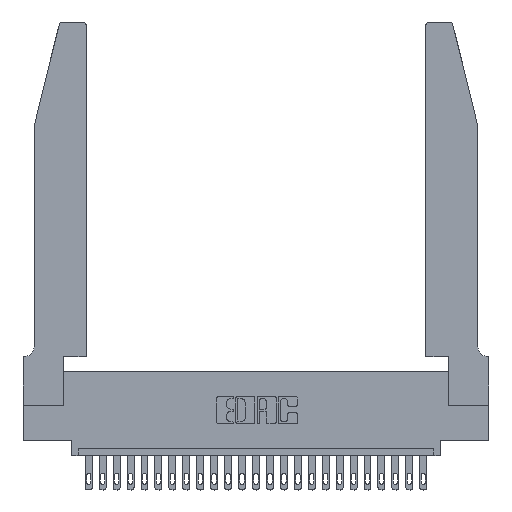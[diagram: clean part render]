
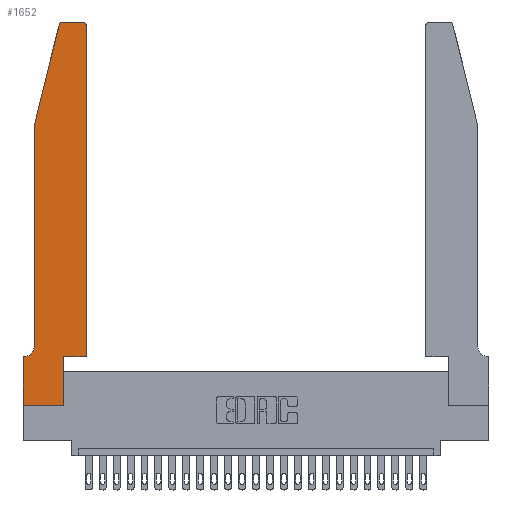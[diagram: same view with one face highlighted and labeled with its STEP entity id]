
A CAD part, top view. The second image highlights one B-rep face of the part: STEP entity #1652.
In plain terms, the highlighted planar face has unit normal (0, 0, 1).
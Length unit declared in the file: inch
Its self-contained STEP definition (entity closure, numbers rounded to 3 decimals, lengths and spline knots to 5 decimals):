
#261 = CIRCLE ( 'NONE', #6762, 0.03 ) ;
#821 = EDGE_CURVE ( 'NONE', #6447, #13358, #22657, .T. ) ;
#1014 = DIRECTION ( 'NONE',  ( 0., 0., 1. ) ) ;
#1505 = VECTOR ( 'NONE', #7983, 39.37008 ) ;
#1580 = CIRCLE ( 'NONE', #14817, 0.03 ) ;
#1652 = ADVANCED_FACE ( 'NONE', ( #4188 ), #17219, .T. ) ;
#2167 = EDGE_LOOP ( 'NONE', ( #10578, #9773, #19002, #25920, #12901, #23125, #11409, #9673, #17620, #21847, #14059, #13561 ) ) ;
#2606 = DIRECTION ( 'NONE',  ( 1., 0., 0. ) ) ;
#2897 = CARTESIAN_POINT ( 'NONE',  ( 0., 0., 0.37 ) ) ;
#3055 = CARTESIAN_POINT ( 'NONE',  ( 0.4205, 2.72, 0.37 ) ) ;
#3140 = CIRCLE ( 'NONE', #5419, 0.07 ) ;
#3270 = EDGE_CURVE ( 'NONE', #13358, #5715, #3789, .T. ) ;
#3565 = DIRECTION ( 'NONE',  ( 0., 1., 0. ) ) ;
#3789 = LINE ( 'NONE', #7729, #19756 ) ;
#3829 = CARTESIAN_POINT ( 'NONE',  ( 0.2865, 0.35, 0.37 ) ) ;
#4188 = FACE_OUTER_BOUND ( 'NONE', #2167, .T. ) ;
#4332 = VECTOR ( 'NONE', #14725, 39.37008 ) ;
#4413 = VECTOR ( 'NONE', #21077, 39.37008 ) ;
#4727 = CARTESIAN_POINT ( 'NONE',  ( 0.284, 2.72, 0.37 ) ) ;
#5323 = DIRECTION ( 'NONE',  ( 1., 0., 0. ) ) ;
#5361 = VERTEX_POINT ( 'NONE', #11329 ) ;
#5419 = AXIS2_PLACEMENT_3D ( 'NONE', #11504, #15531, #23649 ) ;
#5587 = CARTESIAN_POINT ( 'NONE',  ( 0.2865, 0.35, 0.37 ) ) ;
#5715 = VERTEX_POINT ( 'NONE', #2897 ) ;
#6447 = VERTEX_POINT ( 'NONE', #9329 ) ;
#6762 = AXIS2_PLACEMENT_3D ( 'NONE', #3055, #1014, #6830 ) ;
#6830 = DIRECTION ( 'NONE',  ( 1., 0., 0. ) ) ;
#7107 = VERTEX_POINT ( 'NONE', #3829 ) ;
#7338 = VECTOR ( 'NONE', #11303, 39.37008 ) ;
#7363 = EDGE_CURVE ( 'NONE', #20964, #15903, #7788, .T. ) ;
#7438 = EDGE_CURVE ( 'NONE', #7611, #19793, #16521, .T. ) ;
#7512 = CARTESIAN_POINT ( 'NONE',  ( 0.0755, 2., 0.37 ) ) ;
#7611 = VERTEX_POINT ( 'NONE', #14426 ) ;
#7729 = CARTESIAN_POINT ( 'NONE',  ( 0., 0., 0.37 ) ) ;
#7788 = LINE ( 'NONE', #7512, #21860 ) ;
#7983 = DIRECTION ( 'NONE',  ( -0.239, -0.971, 0. ) ) ;
#9158 = AXIS2_PLACEMENT_3D ( 'NONE', #17046, #18964, #5323 ) ;
#9186 = LINE ( 'NONE', #11436, #20135 ) ;
#9329 = CARTESIAN_POINT ( 'NONE',  ( 0.0055, 0.35, 0.37 ) ) ;
#9546 = VERTEX_POINT ( 'NONE', #12481 ) ;
#9673 = ORIENTED_EDGE ( 'NONE', *, *, #23711, .T. ) ;
#9740 = LINE ( 'NONE', #12981, #4413 ) ;
#9773 = ORIENTED_EDGE ( 'NONE', *, *, #23526, .T. ) ;
#10578 = ORIENTED_EDGE ( 'NONE', *, *, #7438, .T. ) ;
#11303 = DIRECTION ( 'NONE',  ( -1., 0., 0. ) ) ;
#11329 = CARTESIAN_POINT ( 'NONE',  ( 0.4505, 2.72, 0.37 ) ) ;
#11409 = ORIENTED_EDGE ( 'NONE', *, *, #3270, .T. ) ;
#11436 = CARTESIAN_POINT ( 'NONE',  ( 0.4505, 0.35, 0.37 ) ) ;
#11504 = CARTESIAN_POINT ( 'NONE',  ( 0.0055, 0.42, 0.37 ) ) ;
#11506 = DIRECTION ( 'NONE',  ( 0., -1., 0. ) ) ;
#11723 = VECTOR ( 'NONE', #13711, 39.37008 ) ;
#12037 = LINE ( 'NONE', #15767, #11723 ) ;
#12481 = CARTESIAN_POINT ( 'NONE',  ( 0.4505, 0.35, 0.37 ) ) ;
#12506 = CARTESIAN_POINT ( 'NONE',  ( 0.0755, 0.35, 0.37 ) ) ;
#12868 = EDGE_CURVE ( 'NONE', #9546, #5361, #9186, .T. ) ;
#12901 = ORIENTED_EDGE ( 'NONE', *, *, #24357, .T. ) ;
#12981 = CARTESIAN_POINT ( 'NONE',  ( 0., 0., 0.37 ) ) ;
#13358 = VERTEX_POINT ( 'NONE', #21281 ) ;
#13403 = DIRECTION ( 'NONE',  ( 0., 1., 0. ) ) ;
#13561 = ORIENTED_EDGE ( 'NONE', *, *, #23752, .T. ) ;
#13711 = DIRECTION ( 'NONE',  ( 1., 0., 0. ) ) ;
#14059 = ORIENTED_EDGE ( 'NONE', *, *, #12868, .T. ) ;
#14117 = VERTEX_POINT ( 'NONE', #20324 ) ;
#14426 = CARTESIAN_POINT ( 'NONE',  ( 0.4205, 2.75, 0.37 ) ) ;
#14725 = DIRECTION ( 'NONE',  ( -1., 0., 0. ) ) ;
#14817 = AXIS2_PLACEMENT_3D ( 'NONE', #4727, #20728, #2606 ) ;
#14819 = VERTEX_POINT ( 'NONE', #21342 ) ;
#15143 = CARTESIAN_POINT ( 'NONE',  ( 0.2605, 2.75, 0.37 ) ) ;
#15531 = DIRECTION ( 'NONE',  ( 0., 0., -1. ) ) ;
#15767 = CARTESIAN_POINT ( 'NONE',  ( 0.4505, 0.35, 0.37 ) ) ;
#15842 = CARTESIAN_POINT ( 'NONE',  ( 0.0755, 2., 0.37 ) ) ;
#15903 = VERTEX_POINT ( 'NONE', #24237 ) ;
#16521 = LINE ( 'NONE', #15143, #4332 ) ;
#16749 = CARTESIAN_POINT ( 'NONE',  ( 0.284, 2.75, 0.37 ) ) ;
#17046 = CARTESIAN_POINT ( 'NONE',  ( 0., 0.35, 0.37 ) ) ;
#17219 = PLANE ( 'NONE',  #9158 ) ;
#17440 = DIRECTION ( 'NONE',  ( 0., -1., 0. ) ) ;
#17620 = ORIENTED_EDGE ( 'NONE', *, *, #23820, .T. ) ;
#18964 = DIRECTION ( 'NONE',  ( 0., 0., 1. ) ) ;
#18995 = EDGE_CURVE ( 'NONE', #7107, #9546, #12037, .T. ) ;
#19002 = ORIENTED_EDGE ( 'NONE', *, *, #25078, .T. ) ;
#19756 = VECTOR ( 'NONE', #17440, 39.37008 ) ;
#19793 = VERTEX_POINT ( 'NONE', #16749 ) ;
#20135 = VECTOR ( 'NONE', #3565, 39.37008 ) ;
#20324 = CARTESIAN_POINT ( 'NONE',  ( 0.25487, 2.72718, 0.37 ) ) ;
#20548 = CARTESIAN_POINT ( 'NONE',  ( 0.0755, 2., 0.37 ) ) ;
#20728 = DIRECTION ( 'NONE',  ( 0., 0., 1. ) ) ;
#20964 = VERTEX_POINT ( 'NONE', #20548 ) ;
#21077 = DIRECTION ( 'NONE',  ( 1., 0., 0. ) ) ;
#21281 = CARTESIAN_POINT ( 'NONE',  ( 0., 0.35, 0.37 ) ) ;
#21342 = CARTESIAN_POINT ( 'NONE',  ( 0.2865, 0., 0.37 ) ) ;
#21847 = ORIENTED_EDGE ( 'NONE', *, *, #18995, .T. ) ;
#21860 = VECTOR ( 'NONE', #11506, 39.37008 ) ;
#22236 = LINE ( 'NONE', #5587, #25011 ) ;
#22487 = LINE ( 'NONE', #15842, #1505 ) ;
#22657 = LINE ( 'NONE', #12506, #7338 ) ;
#23125 = ORIENTED_EDGE ( 'NONE', *, *, #821, .T. ) ;
#23526 = EDGE_CURVE ( 'NONE', #19793, #14117, #1580, .T. ) ;
#23649 = DIRECTION ( 'NONE',  ( -1., 0., 0. ) ) ;
#23711 = EDGE_CURVE ( 'NONE', #5715, #14819, #9740, .T. ) ;
#23752 = EDGE_CURVE ( 'NONE', #5361, #7611, #261, .T. ) ;
#23820 = EDGE_CURVE ( 'NONE', #14819, #7107, #22236, .T. ) ;
#24237 = CARTESIAN_POINT ( 'NONE',  ( 0.0755, 0.42, 0.37 ) ) ;
#24357 = EDGE_CURVE ( 'NONE', #15903, #6447, #3140, .T. ) ;
#25011 = VECTOR ( 'NONE', #13403, 39.37008 ) ;
#25078 = EDGE_CURVE ( 'NONE', #14117, #20964, #22487, .T. ) ;
#25920 = ORIENTED_EDGE ( 'NONE', *, *, #7363, .T. ) ;
